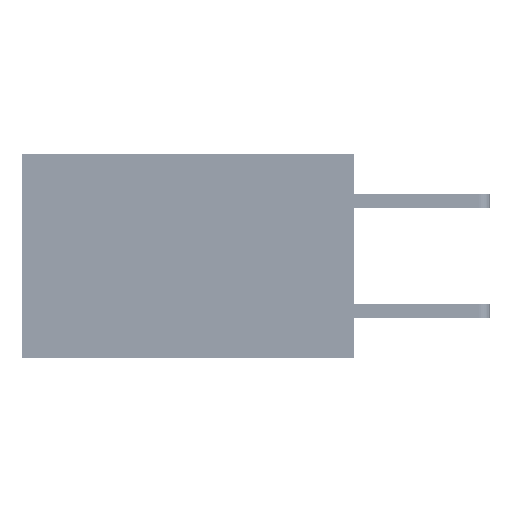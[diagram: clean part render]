
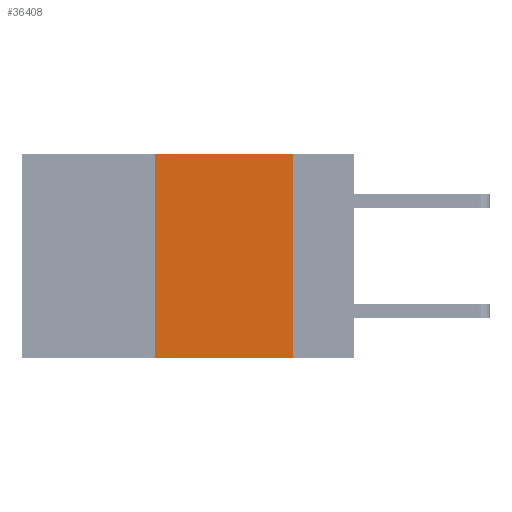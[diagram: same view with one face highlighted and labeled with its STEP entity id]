
A CAD part, left-side view. The second image highlights one B-rep face of the part: STEP entity #36408.
In plain terms, the highlighted planar face has unit normal (-1, 0, 0).
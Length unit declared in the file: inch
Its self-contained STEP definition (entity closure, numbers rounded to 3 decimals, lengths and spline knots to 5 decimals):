
#878 = DIRECTION ( 'NONE',  ( 0., -1., 0. ) ) ;
#2226 = ORIENTED_EDGE ( 'NONE', *, *, #36196, .F. ) ;
#2648 = CARTESIAN_POINT ( 'NONE',  ( 0., 0.36, 0. ) ) ;
#4379 = EDGE_CURVE ( 'NONE', #21762, #35680, #34056, .T. ) ;
#4433 = ORIENTED_EDGE ( 'NONE', *, *, #26323, .T. ) ;
#4736 = AXIS2_PLACEMENT_3D ( 'NONE', #38352, #45541, #31591 ) ;
#4752 = LINE ( 'NONE', #15671, #23395 ) ;
#4980 = DIRECTION ( 'NONE',  ( 0., -1., 0. ) ) ;
#9162 = LINE ( 'NONE', #2648, #40001 ) ;
#10206 = CARTESIAN_POINT ( 'NONE',  ( 0., 0.36, 0. ) ) ;
#11865 = CARTESIAN_POINT ( 'NONE',  ( 0., 0.11, 0. ) ) ;
#15671 = CARTESIAN_POINT ( 'NONE',  ( 0., 0.6, 0. ) ) ;
#15761 = ORIENTED_EDGE ( 'NONE', *, *, #44142, .F. ) ;
#20659 = PLANE ( 'NONE',  #4736 ) ;
#21079 = CARTESIAN_POINT ( 'NONE',  ( 0., 0.36, -0.37 ) ) ;
#21762 = VERTEX_POINT ( 'NONE', #11865 ) ;
#23395 = VECTOR ( 'NONE', #4980, 39.37008 ) ;
#23583 = CARTESIAN_POINT ( 'NONE',  ( 0., 0.11, 0. ) ) ;
#23854 = VECTOR ( 'NONE', #878, 39.37008 ) ;
#24141 = FACE_OUTER_BOUND ( 'NONE', #35904, .T. ) ;
#26323 = EDGE_CURVE ( 'NONE', #45637, #35680, #29027, .T. ) ;
#28164 = ORIENTED_EDGE ( 'NONE', *, *, #4379, .F. ) ;
#29027 = LINE ( 'NONE', #35771, #23854 ) ;
#29139 = VERTEX_POINT ( 'NONE', #10206 ) ;
#30803 = DIRECTION ( 'NONE',  ( 0., 0., -1. ) ) ;
#31591 = DIRECTION ( 'NONE',  ( 0., 0., -1. ) ) ;
#34056 = LINE ( 'NONE', #23583, #35244 ) ;
#35244 = VECTOR ( 'NONE', #30803, 39.37008 ) ;
#35680 = VERTEX_POINT ( 'NONE', #45253 ) ;
#35771 = CARTESIAN_POINT ( 'NONE',  ( 0., 0.6, -0.37 ) ) ;
#35904 = EDGE_LOOP ( 'NONE', ( #28164, #2226, #15761, #4433 ) ) ;
#36196 = EDGE_CURVE ( 'NONE', #29139, #21762, #4752, .T. ) ;
#36408 = ADVANCED_FACE ( 'NONE', ( #24141 ), #20659, .F. ) ;
#38244 = DIRECTION ( 'NONE',  ( 0., 0., 1. ) ) ;
#38352 = CARTESIAN_POINT ( 'NONE',  ( 0., 0.6, 0. ) ) ;
#40001 = VECTOR ( 'NONE', #38244, 39.37008 ) ;
#44142 = EDGE_CURVE ( 'NONE', #45637, #29139, #9162, .T. ) ;
#45253 = CARTESIAN_POINT ( 'NONE',  ( 0., 0.11, -0.37 ) ) ;
#45541 = DIRECTION ( 'NONE',  ( 1., 0., 0. ) ) ;
#45637 = VERTEX_POINT ( 'NONE', #21079 ) ;
